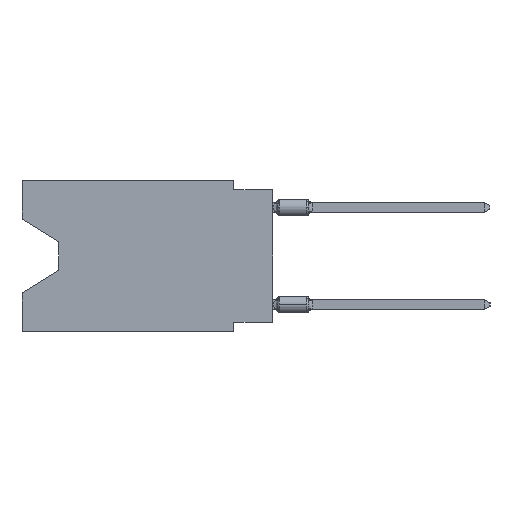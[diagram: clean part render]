
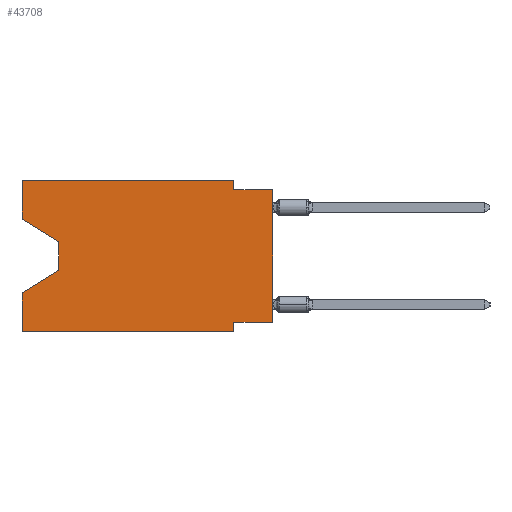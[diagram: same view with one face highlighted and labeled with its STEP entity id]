
A CAD part, left-side view. The second image highlights one B-rep face of the part: STEP entity #43708.
In plain terms, the highlighted planar face has unit normal (-1, 0, 0).
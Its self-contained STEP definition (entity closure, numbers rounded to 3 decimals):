
#501 = VERTEX_POINT ( 'NONE', #46293 ) ;
#1178 = ORIENTED_EDGE ( 'NONE', *, *, #2917, .F. ) ;
#1278 = VECTOR ( 'NONE', #38557, 1000. ) ;
#1370 = VECTOR ( 'NONE', #57189, 1000. ) ;
#2421 = ORIENTED_EDGE ( 'NONE', *, *, #13537, .F. ) ;
#2864 = CARTESIAN_POINT ( 'NONE',  ( 0., 16.383, 0. ) ) ;
#2917 = EDGE_CURVE ( 'NONE', #27867, #14447, #54608, .T. ) ;
#3132 = DIRECTION ( 'NONE',  ( 0., -0.855, -0.519 ) ) ;
#3305 = LINE ( 'NONE', #20834, #37610 ) ;
#3314 = CARTESIAN_POINT ( 'NONE',  ( 0., 16.383, -9.906 ) ) ;
#4792 = CARTESIAN_POINT ( 'NONE',  ( 0., 16.383, 0. ) ) ;
#4861 = VECTOR ( 'NONE', #42129, 1000. ) ;
#5740 = ORIENTED_EDGE ( 'NONE', *, *, #55698, .T. ) ;
#6333 = CARTESIAN_POINT ( 'NONE',  ( 0., 16.383, 0. ) ) ;
#6483 = VERTEX_POINT ( 'NONE', #34520 ) ;
#6593 = LINE ( 'NONE', #21197, #22725 ) ;
#7895 = ORIENTED_EDGE ( 'NONE', *, *, #43452, .F. ) ;
#8119 = LINE ( 'NONE', #43539, #9231 ) ;
#9231 = VECTOR ( 'NONE', #57550, 1000. ) ;
#10226 = DIRECTION ( 'NONE',  ( 0., 0., -1. ) ) ;
#10299 = CARTESIAN_POINT ( 'NONE',  ( 0., 2.54, 0. ) ) ;
#11582 = ORIENTED_EDGE ( 'NONE', *, *, #26602, .F. ) ;
#11722 = VERTEX_POINT ( 'NONE', #21056 ) ;
#12937 = CARTESIAN_POINT ( 'NONE',  ( 0., 13.97, -5.893 ) ) ;
#13377 = CARTESIAN_POINT ( 'NONE',  ( 0., 16.383, 0. ) ) ;
#13537 = EDGE_CURVE ( 'NONE', #18543, #20733, #24361, .T. ) ;
#13972 = VERTEX_POINT ( 'NONE', #20126 ) ;
#14187 = EDGE_CURVE ( 'NONE', #13972, #49883, #8119, .T. ) ;
#14447 = VERTEX_POINT ( 'NONE', #20350 ) ;
#15083 = DIRECTION ( 'NONE',  ( 0., -1., 0. ) ) ;
#17915 = VECTOR ( 'NONE', #3132, 1000. ) ;
#18372 = CARTESIAN_POINT ( 'NONE',  ( 0., 2.54, -0.635 ) ) ;
#18543 = VERTEX_POINT ( 'NONE', #18372 ) ;
#20013 = EDGE_CURVE ( 'NONE', #6483, #13972, #29164, .T. ) ;
#20126 = CARTESIAN_POINT ( 'NONE',  ( 0., 13.97, -4.013 ) ) ;
#20350 = CARTESIAN_POINT ( 'NONE',  ( 0., 2.54, 0. ) ) ;
#20409 = LINE ( 'NONE', #2864, #1278 ) ;
#20506 = ORIENTED_EDGE ( 'NONE', *, *, #14187, .T. ) ;
#20559 = CARTESIAN_POINT ( 'NONE',  ( 0., 13.97, -5.893 ) ) ;
#20733 = VERTEX_POINT ( 'NONE', #50890 ) ;
#20834 = CARTESIAN_POINT ( 'NONE',  ( 0., 0., -9.271 ) ) ;
#21056 = CARTESIAN_POINT ( 'NONE',  ( 0., 2.54, -9.271 ) ) ;
#21197 = CARTESIAN_POINT ( 'NONE',  ( 0., 16.383, -9.906 ) ) ;
#21501 = VERTEX_POINT ( 'NONE', #48171 ) ;
#21942 = EDGE_CURVE ( 'NONE', #11722, #21501, #39629, .T. ) ;
#22463 = EDGE_CURVE ( 'NONE', #55770, #57612, #20409, .T. ) ;
#22725 = VECTOR ( 'NONE', #52786, 1000. ) ;
#22860 = ORIENTED_EDGE ( 'NONE', *, *, #22463, .F. ) ;
#23100 = EDGE_CURVE ( 'NONE', #6483, #27867, #39642, .T. ) ;
#24361 = LINE ( 'NONE', #24659, #32422 ) ;
#24515 = ORIENTED_EDGE ( 'NONE', *, *, #20013, .T. ) ;
#24659 = CARTESIAN_POINT ( 'NONE',  ( 0., 0., -0.635 ) ) ;
#25062 = EDGE_LOOP ( 'NONE', ( #24515, #20506, #5740, #22860, #54331, #48583, #11582, #29001, #2421, #7895, #1178, #56001 ) ) ;
#26602 = EDGE_CURVE ( 'NONE', #501, #11722, #3305, .T. ) ;
#27867 = VERTEX_POINT ( 'NONE', #13377 ) ;
#29001 = ORIENTED_EDGE ( 'NONE', *, *, #46171, .T. ) ;
#29038 = DIRECTION ( 'NONE',  ( 0., -1., 0. ) ) ;
#29164 = LINE ( 'NONE', #29462, #17915 ) ;
#29462 = CARTESIAN_POINT ( 'NONE',  ( 0., 16.383, -2.546 ) ) ;
#31316 = CARTESIAN_POINT ( 'NONE',  ( 0., 16.383, 0. ) ) ;
#32177 = CARTESIAN_POINT ( 'NONE',  ( 0., 16.383, -7.36 ) ) ;
#32422 = VECTOR ( 'NONE', #29038, 1000. ) ;
#33348 = LINE ( 'NONE', #50018, #4861 ) ;
#34520 = CARTESIAN_POINT ( 'NONE',  ( 0., 16.383, -2.546 ) ) ;
#35704 = FACE_OUTER_BOUND ( 'NONE', #25062, .T. ) ;
#37610 = VECTOR ( 'NONE', #38710, 1000. ) ;
#38557 = DIRECTION ( 'NONE',  ( 0., 0., 1. ) ) ;
#38710 = DIRECTION ( 'NONE',  ( 0., 1., 0. ) ) ;
#39064 = DIRECTION ( 'NONE',  ( 0., 0., -1. ) ) ;
#39629 = LINE ( 'NONE', #48103, #44212 ) ;
#39642 = LINE ( 'NONE', #4792, #1370 ) ;
#42129 = DIRECTION ( 'NONE',  ( 0., 0., 1. ) ) ;
#42737 = VECTOR ( 'NONE', #45981, 1000. ) ;
#43452 = EDGE_CURVE ( 'NONE', #14447, #18543, #50368, .T. ) ;
#43539 = CARTESIAN_POINT ( 'NONE',  ( 0., 13.97, -4.013 ) ) ;
#43708 = ADVANCED_FACE ( 'NONE', ( #35704 ), #53530, .F. ) ;
#44212 = VECTOR ( 'NONE', #39064, 1000. ) ;
#45981 = DIRECTION ( 'NONE',  ( 0., 0., -1. ) ) ;
#46171 = EDGE_CURVE ( 'NONE', #501, #20733, #33348, .T. ) ;
#46293 = CARTESIAN_POINT ( 'NONE',  ( 0., 0., -9.271 ) ) ;
#47189 = DIRECTION ( 'NONE',  ( 0., 0.855, -0.519 ) ) ;
#48103 = CARTESIAN_POINT ( 'NONE',  ( 0., 2.54, -9.906 ) ) ;
#48162 = EDGE_CURVE ( 'NONE', #55770, #21501, #6593, .T. ) ;
#48171 = CARTESIAN_POINT ( 'NONE',  ( 0., 2.54, -9.906 ) ) ;
#48375 = VECTOR ( 'NONE', #47189, 1000. ) ;
#48583 = ORIENTED_EDGE ( 'NONE', *, *, #21942, .F. ) ;
#49136 = DIRECTION ( 'NONE',  ( 1., 0., 0. ) ) ;
#49883 = VERTEX_POINT ( 'NONE', #12937 ) ;
#50018 = CARTESIAN_POINT ( 'NONE',  ( 0., 0., 0. ) ) ;
#50368 = LINE ( 'NONE', #10299, #42737 ) ;
#50890 = CARTESIAN_POINT ( 'NONE',  ( 0., 0., -0.635 ) ) ;
#51287 = LINE ( 'NONE', #20559, #48375 ) ;
#52035 = AXIS2_PLACEMENT_3D ( 'NONE', #31316, #49136, #10226 ) ;
#52786 = DIRECTION ( 'NONE',  ( 0., -1., 0. ) ) ;
#53530 = PLANE ( 'NONE',  #52035 ) ;
#54331 = ORIENTED_EDGE ( 'NONE', *, *, #48162, .T. ) ;
#54608 = LINE ( 'NONE', #6333, #54629 ) ;
#54629 = VECTOR ( 'NONE', #15083, 1000. ) ;
#55698 = EDGE_CURVE ( 'NONE', #49883, #57612, #51287, .T. ) ;
#55770 = VERTEX_POINT ( 'NONE', #3314 ) ;
#56001 = ORIENTED_EDGE ( 'NONE', *, *, #23100, .F. ) ;
#57189 = DIRECTION ( 'NONE',  ( 0., 0., 1. ) ) ;
#57550 = DIRECTION ( 'NONE',  ( 0., 0., -1. ) ) ;
#57612 = VERTEX_POINT ( 'NONE', #32177 ) ;
